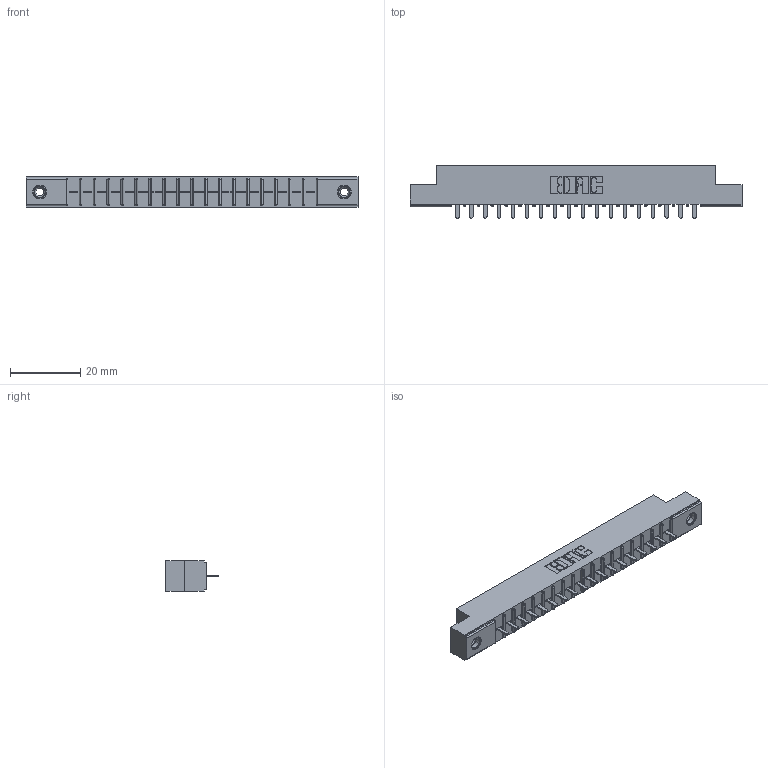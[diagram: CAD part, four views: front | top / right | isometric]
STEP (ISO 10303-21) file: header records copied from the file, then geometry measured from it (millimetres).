
FILE_DESCRIPTION (( 'STEP AP203' ), '1' );
FILE_NAME ('316-018-421-108.STEP', '2020-09-22T18:49:33', ( '' ), ( '' ), 'SwSTEP 2.0', 'SolidWorks 2020', '' );
FILE_SCHEMA (( 'CONFIG_CONTROL_DESIGN' ));
Length unit declared in the file: inch
Products named in the file (4): 345-250-001_345-250-003-102; 306 Part_.156 Dia; 316-018-421-108; 306-290-001_121
Assembly tree (21 placements, depth 2):
  316-018-421-108
    306 Part_.156 Dia
    306-290-001_121  x18
    345-250-001_345-250-003-102  x2
Bounding box: 94.34 x 14.88 x 8.71 mm (x, y, z)
Volume: 6408.5 mm3; surface area: 9239.3 mm2
Topology: 21 solids, 21 shells, 1436 faces, 3998 edges, 2560 vertices
Faces by surface type: plane 946, cylinder 402, sphere 72, cone 12, torus 4
Entity records: 21036 total; most frequent: CARTESIAN_POINT 3508, DIRECTION 3470, ORIENTED_EDGE 3468, EDGE_CURVE 1734, VECTOR 1342, LINE 1342, VERTEX_POINT 1102, AXIS2_PLACEMENT_3D 1064
